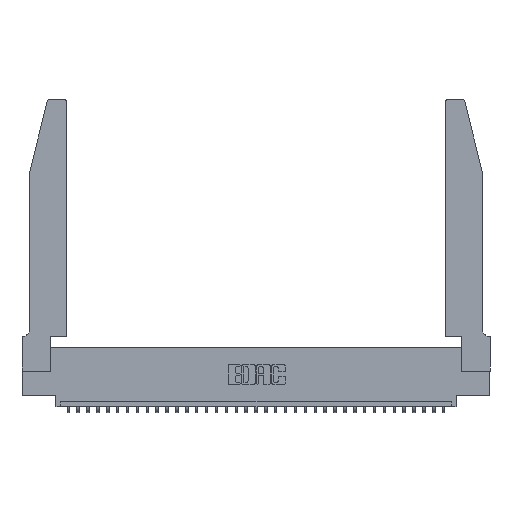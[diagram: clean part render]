
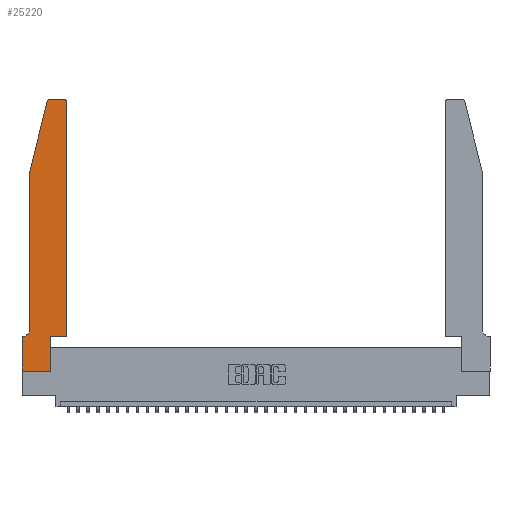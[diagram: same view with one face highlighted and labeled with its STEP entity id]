
A CAD part, top view. The second image highlights one B-rep face of the part: STEP entity #25220.
In plain terms, the highlighted planar face has unit normal (0, 0, 1).
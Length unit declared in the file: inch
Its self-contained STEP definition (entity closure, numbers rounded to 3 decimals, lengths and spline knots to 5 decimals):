
#650 = LINE ( 'NONE', #28347, #24939 ) ;
#816 = EDGE_LOOP ( 'NONE', ( #16437, #26252, #23680, #21651, #10300, #33743, #28262, #32573, #5352, #15199, #33573, #33121 ) ) ;
#1268 = VERTEX_POINT ( 'NONE', #12559 ) ;
#1494 = CARTESIAN_POINT ( 'NONE',  ( 0.4505, 0.35, 0.37 ) ) ;
#1554 = LINE ( 'NONE', #9289, #32546 ) ;
#1859 = CARTESIAN_POINT ( 'NONE',  ( 0.0755, 2., 0.37 ) ) ;
#2008 = EDGE_CURVE ( 'NONE', #32841, #29480, #12408, .T. ) ;
#3615 = CARTESIAN_POINT ( 'NONE',  ( 0., 0., 0.37 ) ) ;
#3903 = AXIS2_PLACEMENT_3D ( 'NONE', #15910, #32197, #34453 ) ;
#4133 = LINE ( 'NONE', #9449, #8276 ) ;
#4865 = VERTEX_POINT ( 'NONE', #13016 ) ;
#5346 = FACE_OUTER_BOUND ( 'NONE', #816, .T. ) ;
#5352 = ORIENTED_EDGE ( 'NONE', *, *, #31417, .T. ) ;
#5873 = CARTESIAN_POINT ( 'NONE',  ( 0.4505, 2.72, 0.37 ) ) ;
#6950 = VERTEX_POINT ( 'NONE', #24639 ) ;
#7078 = LINE ( 'NONE', #12245, #33461 ) ;
#7157 = VERTEX_POINT ( 'NONE', #15181 ) ;
#7507 = DIRECTION ( 'NONE',  ( 1., 0., 0. ) ) ;
#8045 = VERTEX_POINT ( 'NONE', #34527 ) ;
#8276 = VECTOR ( 'NONE', #25219, 39.37008 ) ;
#8406 = DIRECTION ( 'NONE',  ( 1., 0., 0. ) ) ;
#8477 = VECTOR ( 'NONE', #21678, 39.37008 ) ;
#8670 = EDGE_CURVE ( 'NONE', #7157, #14239, #16015, .T. ) ;
#9289 = CARTESIAN_POINT ( 'NONE',  ( 0.4505, 0.35, 0.37 ) ) ;
#9336 = CARTESIAN_POINT ( 'NONE',  ( 0.0755, 0.42, 0.37 ) ) ;
#9449 = CARTESIAN_POINT ( 'NONE',  ( 0.0755, 0.35, 0.37 ) ) ;
#9987 = VERTEX_POINT ( 'NONE', #5873 ) ;
#10300 = ORIENTED_EDGE ( 'NONE', *, *, #2008, .T. ) ;
#10606 = VERTEX_POINT ( 'NONE', #30242 ) ;
#10781 = EDGE_CURVE ( 'NONE', #29480, #8045, #4133, .T. ) ;
#10995 = AXIS2_PLACEMENT_3D ( 'NONE', #16102, #26643, #18758 ) ;
#11653 = EDGE_CURVE ( 'NONE', #14239, #9987, #1554, .T. ) ;
#12059 = EDGE_CURVE ( 'NONE', #8045, #10606, #21204, .T. ) ;
#12245 = CARTESIAN_POINT ( 'NONE',  ( 0.0755, 2., 0.37 ) ) ;
#12408 = CIRCLE ( 'NONE', #3903, 0.07 ) ;
#12559 = CARTESIAN_POINT ( 'NONE',  ( 0.25487, 2.72718, 0.37 ) ) ;
#12702 = DIRECTION ( 'NONE',  ( -0.239, -0.971, 0. ) ) ;
#13016 = CARTESIAN_POINT ( 'NONE',  ( 0.4205, 2.75, 0.37 ) ) ;
#13262 = CARTESIAN_POINT ( 'NONE',  ( 0.0055, 0.35, 0.37 ) ) ;
#13323 = CARTESIAN_POINT ( 'NONE',  ( 0.284, 2.72, 0.37 ) ) ;
#13557 = AXIS2_PLACEMENT_3D ( 'NONE', #13323, #24529, #8406 ) ;
#14239 = VERTEX_POINT ( 'NONE', #1494 ) ;
#14497 = EDGE_CURVE ( 'NONE', #4865, #6950, #34738, .T. ) ;
#14717 = CARTESIAN_POINT ( 'NONE',  ( 0.2605, 2.75, 0.37 ) ) ;
#14839 = DIRECTION ( 'NONE',  ( 1., 0., 0. ) ) ;
#15181 = CARTESIAN_POINT ( 'NONE',  ( 0.2865, 0.35, 0.37 ) ) ;
#15199 = ORIENTED_EDGE ( 'NONE', *, *, #8670, .T. ) ;
#15910 = CARTESIAN_POINT ( 'NONE',  ( 0.0055, 0.42, 0.37 ) ) ;
#16015 = LINE ( 'NONE', #18334, #34496 ) ;
#16102 = CARTESIAN_POINT ( 'NONE',  ( 0., 0.35, 0.37 ) ) ;
#16437 = ORIENTED_EDGE ( 'NONE', *, *, #14497, .T. ) ;
#17954 = AXIS2_PLACEMENT_3D ( 'NONE', #20071, #25820, #14839 ) ;
#18334 = CARTESIAN_POINT ( 'NONE',  ( 0.4505, 0.35, 0.37 ) ) ;
#18758 = DIRECTION ( 'NONE',  ( 1., 0., 0. ) ) ;
#19477 = CARTESIAN_POINT ( 'NONE',  ( 0.2865, 0., 0.37 ) ) ;
#19580 = VECTOR ( 'NONE', #25587, 39.37008 ) ;
#20071 = CARTESIAN_POINT ( 'NONE',  ( 0.4205, 2.72, 0.37 ) ) ;
#21204 = LINE ( 'NONE', #3615, #21585 ) ;
#21449 = LINE ( 'NONE', #26993, #8477 ) ;
#21585 = VECTOR ( 'NONE', #33401, 39.37008 ) ;
#21651 = ORIENTED_EDGE ( 'NONE', *, *, #26874, .T. ) ;
#21678 = DIRECTION ( 'NONE',  ( 0., -1., 0. ) ) ;
#21987 = DIRECTION ( 'NONE',  ( 0., 1., 0. ) ) ;
#23312 = DIRECTION ( 'NONE',  ( 1., 0., 0. ) ) ;
#23680 = ORIENTED_EDGE ( 'NONE', *, *, #29323, .T. ) ;
#24529 = DIRECTION ( 'NONE',  ( 0., 0., 1. ) ) ;
#24639 = CARTESIAN_POINT ( 'NONE',  ( 0.284, 2.75, 0.37 ) ) ;
#24939 = VECTOR ( 'NONE', #23312, 39.37008 ) ;
#25219 = DIRECTION ( 'NONE',  ( -1., 0., 0. ) ) ;
#25220 = ADVANCED_FACE ( 'NONE', ( #5346 ), #31937, .T. ) ;
#25587 = DIRECTION ( 'NONE',  ( -1., 0., 0. ) ) ;
#25820 = DIRECTION ( 'NONE',  ( 0., 0., 1. ) ) ;
#26252 = ORIENTED_EDGE ( 'NONE', *, *, #31824, .T. ) ;
#26543 = VERTEX_POINT ( 'NONE', #1859 ) ;
#26643 = DIRECTION ( 'NONE',  ( 0., 0., 1. ) ) ;
#26874 = EDGE_CURVE ( 'NONE', #26543, #32841, #21449, .T. ) ;
#26993 = CARTESIAN_POINT ( 'NONE',  ( 0.0755, 2., 0.37 ) ) ;
#27114 = EDGE_CURVE ( 'NONE', #9987, #4865, #30210, .T. ) ;
#28262 = ORIENTED_EDGE ( 'NONE', *, *, #12059, .T. ) ;
#28347 = CARTESIAN_POINT ( 'NONE',  ( 0., 0., 0.37 ) ) ;
#29061 = VERTEX_POINT ( 'NONE', #19477 ) ;
#29323 = EDGE_CURVE ( 'NONE', #1268, #26543, #7078, .T. ) ;
#29480 = VERTEX_POINT ( 'NONE', #13262 ) ;
#30210 = CIRCLE ( 'NONE', #17954, 0.03 ) ;
#30242 = CARTESIAN_POINT ( 'NONE',  ( 0., 0., 0.37 ) ) ;
#30850 = LINE ( 'NONE', #32690, #32917 ) ;
#31417 = EDGE_CURVE ( 'NONE', #29061, #7157, #30850, .T. ) ;
#31452 = CIRCLE ( 'NONE', #13557, 0.03 ) ;
#31606 = DIRECTION ( 'NONE',  ( 0., 1., 0. ) ) ;
#31613 = EDGE_CURVE ( 'NONE', #10606, #29061, #650, .T. ) ;
#31824 = EDGE_CURVE ( 'NONE', #6950, #1268, #31452, .T. ) ;
#31937 = PLANE ( 'NONE',  #10995 ) ;
#32197 = DIRECTION ( 'NONE',  ( 0., 0., -1. ) ) ;
#32546 = VECTOR ( 'NONE', #31606, 39.37008 ) ;
#32573 = ORIENTED_EDGE ( 'NONE', *, *, #31613, .T. ) ;
#32690 = CARTESIAN_POINT ( 'NONE',  ( 0.2865, 0.35, 0.37 ) ) ;
#32841 = VERTEX_POINT ( 'NONE', #9336 ) ;
#32917 = VECTOR ( 'NONE', #21987, 39.37008 ) ;
#33121 = ORIENTED_EDGE ( 'NONE', *, *, #27114, .T. ) ;
#33401 = DIRECTION ( 'NONE',  ( 0., -1., 0. ) ) ;
#33461 = VECTOR ( 'NONE', #12702, 39.37008 ) ;
#33573 = ORIENTED_EDGE ( 'NONE', *, *, #11653, .T. ) ;
#33743 = ORIENTED_EDGE ( 'NONE', *, *, #10781, .T. ) ;
#34453 = DIRECTION ( 'NONE',  ( -1., 0., 0. ) ) ;
#34496 = VECTOR ( 'NONE', #7507, 39.37008 ) ;
#34527 = CARTESIAN_POINT ( 'NONE',  ( 0., 0.35, 0.37 ) ) ;
#34738 = LINE ( 'NONE', #14717, #19580 ) ;
